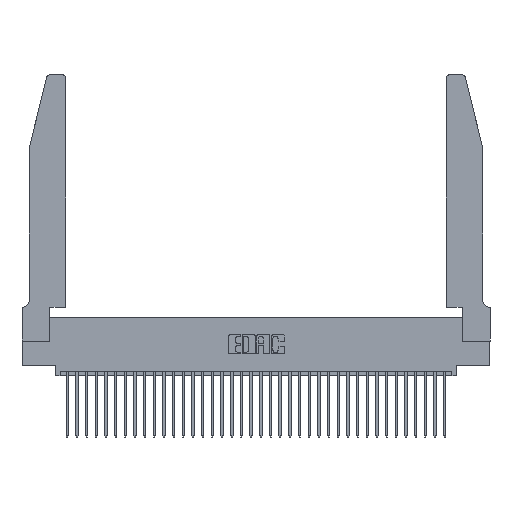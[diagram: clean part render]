
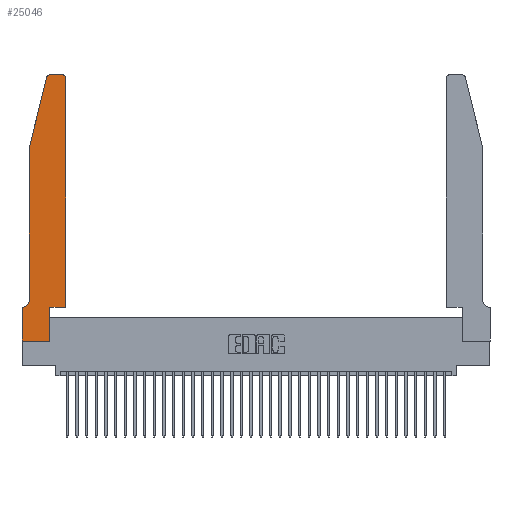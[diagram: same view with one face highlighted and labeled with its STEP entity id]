
A CAD part, top view. The second image highlights one B-rep face of the part: STEP entity #25046.
In plain terms, the highlighted planar face has unit normal (0, 0, 1).
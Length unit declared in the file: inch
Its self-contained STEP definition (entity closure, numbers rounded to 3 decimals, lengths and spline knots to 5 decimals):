
#178 = EDGE_CURVE ( 'NONE', #30445, #33225, #30392, .T. ) ;
#346 = VERTEX_POINT ( 'NONE', #9121 ) ;
#1865 = CARTESIAN_POINT ( 'NONE',  ( 0.2865, 0.35, 0.37 ) ) ;
#1952 = LINE ( 'NONE', #9797, #12078 ) ;
#2117 = AXIS2_PLACEMENT_3D ( 'NONE', #8817, #26039, #9149 ) ;
#2227 = DIRECTION ( 'NONE',  ( 0., 0., -1. ) ) ;
#2455 = VERTEX_POINT ( 'NONE', #12099 ) ;
#2681 = VERTEX_POINT ( 'NONE', #18560 ) ;
#2819 = DIRECTION ( 'NONE',  ( 1., 0., 0. ) ) ;
#3325 = ORIENTED_EDGE ( 'NONE', *, *, #21356, .T. ) ;
#4225 = EDGE_CURVE ( 'NONE', #2455, #2681, #21135, .T. ) ;
#4351 = EDGE_LOOP ( 'NONE', ( #28248, #28048, #23496, #4705, #3325, #15571, #35606, #17407, #35945, #30888, #19974, #20791 ) ) ;
#4361 = PLANE ( 'NONE',  #20121 ) ;
#4705 = ORIENTED_EDGE ( 'NONE', *, *, #25735, .T. ) ;
#4773 = LINE ( 'NONE', #28659, #8772 ) ;
#4800 = CARTESIAN_POINT ( 'NONE',  ( 0.0055, 0.35, 0.37 ) ) ;
#4918 = DIRECTION ( 'NONE',  ( 0., 1., 0. ) ) ;
#5548 = CARTESIAN_POINT ( 'NONE',  ( 0.4505, 2.72, 0.37 ) ) ;
#5593 = CARTESIAN_POINT ( 'NONE',  ( 0.284, 2.72, 0.37 ) ) ;
#5777 = CIRCLE ( 'NONE', #2117, 0.03 ) ;
#6667 = CARTESIAN_POINT ( 'NONE',  ( 0.2865, 0., 0.37 ) ) ;
#6767 = LINE ( 'NONE', #19167, #22716 ) ;
#7383 = VECTOR ( 'NONE', #14149, 39.37008 ) ;
#7831 = VERTEX_POINT ( 'NONE', #15333 ) ;
#8443 = VECTOR ( 'NONE', #15222, 39.37008 ) ;
#8772 = VECTOR ( 'NONE', #14688, 39.37008 ) ;
#8780 = CARTESIAN_POINT ( 'NONE',  ( 0.0755, 2., 0.37 ) ) ;
#8817 = CARTESIAN_POINT ( 'NONE',  ( 0.4205, 2.72, 0.37 ) ) ;
#9121 = CARTESIAN_POINT ( 'NONE',  ( 0.0755, 0.42, 0.37 ) ) ;
#9149 = DIRECTION ( 'NONE',  ( 1., 0., 0. ) ) ;
#9797 = CARTESIAN_POINT ( 'NONE',  ( 0.2865, 0.35, 0.37 ) ) ;
#9943 = CARTESIAN_POINT ( 'NONE',  ( 0.4505, 0.35, 0.37 ) ) ;
#10169 = DIRECTION ( 'NONE',  ( 1., 0., 0. ) ) ;
#10331 = CARTESIAN_POINT ( 'NONE',  ( 0.4505, 0.35, 0.37 ) ) ;
#10782 = DIRECTION ( 'NONE',  ( -1., 0., 0. ) ) ;
#11290 = EDGE_CURVE ( 'NONE', #35891, #30786, #17468, .T. ) ;
#11407 = VECTOR ( 'NONE', #15794, 39.37008 ) ;
#11575 = DIRECTION ( 'NONE',  ( -0.239, -0.971, 0. ) ) ;
#11614 = FACE_OUTER_BOUND ( 'NONE', #4351, .T. ) ;
#12078 = VECTOR ( 'NONE', #18276, 39.37008 ) ;
#12099 = CARTESIAN_POINT ( 'NONE',  ( 0.25487, 2.72718, 0.37 ) ) ;
#13182 = DIRECTION ( 'NONE',  ( 1., 0., 0. ) ) ;
#13269 = DIRECTION ( 'NONE',  ( 0., -1., 0. ) ) ;
#13529 = EDGE_CURVE ( 'NONE', #7831, #15710, #17514, .T. ) ;
#13593 = VECTOR ( 'NONE', #4918, 39.37008 ) ;
#13789 = EDGE_CURVE ( 'NONE', #35664, #35891, #4773, .T. ) ;
#14098 = DIRECTION ( 'NONE',  ( 0., 0., 1. ) ) ;
#14149 = DIRECTION ( 'NONE',  ( 0., -1., 0. ) ) ;
#14688 = DIRECTION ( 'NONE',  ( -1., 0., 0. ) ) ;
#15222 = DIRECTION ( 'NONE',  ( 1., 0., 0. ) ) ;
#15321 = CIRCLE ( 'NONE', #20723, 0.07 ) ;
#15333 = CARTESIAN_POINT ( 'NONE',  ( 0.4205, 2.75, 0.37 ) ) ;
#15489 = EDGE_CURVE ( 'NONE', #15526, #33625, #1952, .T. ) ;
#15526 = VERTEX_POINT ( 'NONE', #6667 ) ;
#15571 = ORIENTED_EDGE ( 'NONE', *, *, #13789, .T. ) ;
#15656 = CARTESIAN_POINT ( 'NONE',  ( 0., 0., 0.37 ) ) ;
#15710 = VERTEX_POINT ( 'NONE', #30342 ) ;
#15794 = DIRECTION ( 'NONE',  ( -1., 0., 0. ) ) ;
#17238 = CIRCLE ( 'NONE', #28182, 0.03 ) ;
#17407 = ORIENTED_EDGE ( 'NONE', *, *, #29375, .T. ) ;
#17468 = LINE ( 'NONE', #25391, #7383 ) ;
#17514 = LINE ( 'NONE', #23129, #11407 ) ;
#18276 = DIRECTION ( 'NONE',  ( 0., 1., 0. ) ) ;
#18560 = CARTESIAN_POINT ( 'NONE',  ( 0.0755, 2., 0.37 ) ) ;
#19167 = CARTESIAN_POINT ( 'NONE',  ( 0.0755, 2., 0.37 ) ) ;
#19887 = VECTOR ( 'NONE', #11575, 39.37008 ) ;
#19974 = ORIENTED_EDGE ( 'NONE', *, *, #178, .T. ) ;
#20121 = AXIS2_PLACEMENT_3D ( 'NONE', #26849, #27113, #10169 ) ;
#20263 = EDGE_CURVE ( 'NONE', #33225, #7831, #5777, .T. ) ;
#20723 = AXIS2_PLACEMENT_3D ( 'NONE', #32587, #2227, #10782 ) ;
#20791 = ORIENTED_EDGE ( 'NONE', *, *, #20263, .T. ) ;
#21135 = LINE ( 'NONE', #8780, #19887 ) ;
#21356 = EDGE_CURVE ( 'NONE', #346, #35664, #15321, .T. ) ;
#22716 = VECTOR ( 'NONE', #13269, 39.37008 ) ;
#22949 = LINE ( 'NONE', #9943, #31750 ) ;
#23129 = CARTESIAN_POINT ( 'NONE',  ( 0.2605, 2.75, 0.37 ) ) ;
#23496 = ORIENTED_EDGE ( 'NONE', *, *, #4225, .T. ) ;
#23827 = LINE ( 'NONE', #31910, #8443 ) ;
#25046 = ADVANCED_FACE ( 'NONE', ( #11614 ), #4361, .T. ) ;
#25288 = CARTESIAN_POINT ( 'NONE',  ( 0.4505, 0.35, 0.37 ) ) ;
#25391 = CARTESIAN_POINT ( 'NONE',  ( 0., 0., 0.37 ) ) ;
#25735 = EDGE_CURVE ( 'NONE', #2681, #346, #6767, .T. ) ;
#26039 = DIRECTION ( 'NONE',  ( 0., 0., 1. ) ) ;
#26849 = CARTESIAN_POINT ( 'NONE',  ( 0., 0.35, 0.37 ) ) ;
#27113 = DIRECTION ( 'NONE',  ( 0., 0., 1. ) ) ;
#28048 = ORIENTED_EDGE ( 'NONE', *, *, #32510, .T. ) ;
#28182 = AXIS2_PLACEMENT_3D ( 'NONE', #5593, #14098, #2819 ) ;
#28248 = ORIENTED_EDGE ( 'NONE', *, *, #13529, .T. ) ;
#28281 = CARTESIAN_POINT ( 'NONE',  ( 0., 0.35, 0.37 ) ) ;
#28659 = CARTESIAN_POINT ( 'NONE',  ( 0.0755, 0.35, 0.37 ) ) ;
#29375 = EDGE_CURVE ( 'NONE', #30786, #15526, #23827, .T. ) ;
#29534 = EDGE_CURVE ( 'NONE', #33625, #30445, #22949, .T. ) ;
#30342 = CARTESIAN_POINT ( 'NONE',  ( 0.284, 2.75, 0.37 ) ) ;
#30392 = LINE ( 'NONE', #10331, #13593 ) ;
#30445 = VERTEX_POINT ( 'NONE', #25288 ) ;
#30786 = VERTEX_POINT ( 'NONE', #15656 ) ;
#30888 = ORIENTED_EDGE ( 'NONE', *, *, #29534, .T. ) ;
#31750 = VECTOR ( 'NONE', #13182, 39.37008 ) ;
#31910 = CARTESIAN_POINT ( 'NONE',  ( 0., 0., 0.37 ) ) ;
#32510 = EDGE_CURVE ( 'NONE', #15710, #2455, #17238, .T. ) ;
#32587 = CARTESIAN_POINT ( 'NONE',  ( 0.0055, 0.42, 0.37 ) ) ;
#33225 = VERTEX_POINT ( 'NONE', #5548 ) ;
#33625 = VERTEX_POINT ( 'NONE', #1865 ) ;
#35606 = ORIENTED_EDGE ( 'NONE', *, *, #11290, .T. ) ;
#35664 = VERTEX_POINT ( 'NONE', #4800 ) ;
#35891 = VERTEX_POINT ( 'NONE', #28281 ) ;
#35945 = ORIENTED_EDGE ( 'NONE', *, *, #15489, .T. ) ;
